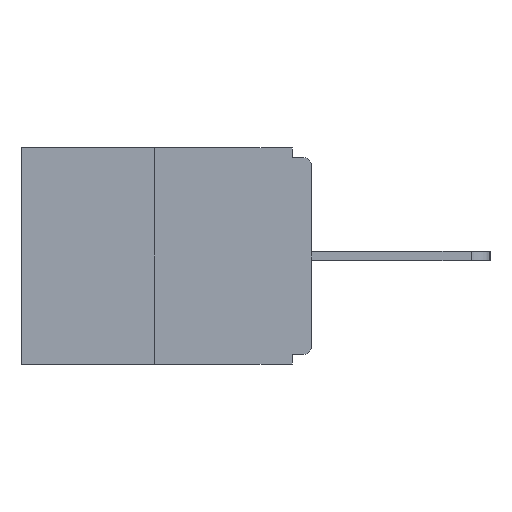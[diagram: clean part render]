
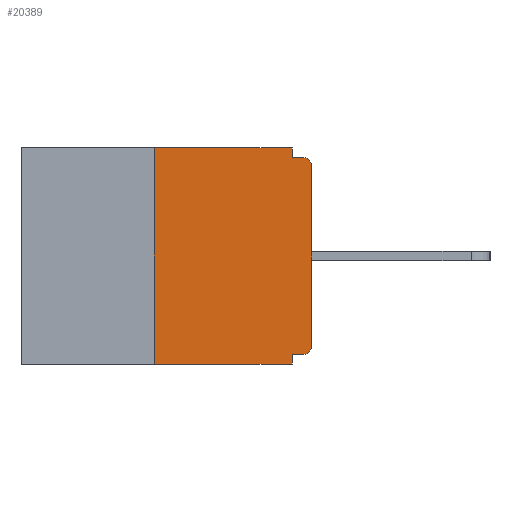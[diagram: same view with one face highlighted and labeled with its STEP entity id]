
A CAD part, left-side view. The second image highlights one B-rep face of the part: STEP entity #20389.
In plain terms, the highlighted planar face has unit normal (-1, 0, 0).
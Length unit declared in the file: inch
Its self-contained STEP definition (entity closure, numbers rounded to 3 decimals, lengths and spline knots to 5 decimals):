
#1220 = VERTEX_POINT ( 'NONE', #17548 ) ;
#1407 = ORIENTED_EDGE ( 'NONE', *, *, #8401, .F. ) ;
#2063 = VERTEX_POINT ( 'NONE', #13509 ) ;
#2719 = VERTEX_POINT ( 'NONE', #18350 ) ;
#2944 = LINE ( 'NONE', #21198, #15774 ) ;
#2949 = DIRECTION ( 'NONE',  ( 0., 0., -1. ) ) ;
#3166 = LINE ( 'NONE', #19771, #17741 ) ;
#3324 = ORIENTED_EDGE ( 'NONE', *, *, #24684, .T. ) ;
#3380 = VERTEX_POINT ( 'NONE', #17262 ) ;
#3836 = PLANE ( 'NONE',  #10884 ) ;
#3865 = EDGE_CURVE ( 'NONE', #14856, #2719, #7147, .T. ) ;
#3969 = DIRECTION ( 'NONE',  ( 0., 0., -1. ) ) ;
#4309 = ORIENTED_EDGE ( 'NONE', *, *, #19632, .F. ) ;
#4408 = ORIENTED_EDGE ( 'NONE', *, *, #24404, .F. ) ;
#4678 = ORIENTED_EDGE ( 'NONE', *, *, #18604, .T. ) ;
#4905 = EDGE_CURVE ( 'NONE', #25087, #2719, #6187, .T. ) ;
#5219 = CARTESIAN_POINT ( 'NONE',  ( 0., 0.46, -0.343 ) ) ;
#6042 = DIRECTION ( 'NONE',  ( 0., 0., -1. ) ) ;
#6187 = LINE ( 'NONE', #24744, #19997 ) ;
#6413 = ORIENTED_EDGE ( 'NONE', *, *, #9980, .F. ) ;
#7147 = LINE ( 'NONE', #5219, #26081 ) ;
#7613 = LINE ( 'NONE', #7879, #17955 ) ;
#7879 = CARTESIAN_POINT ( 'NONE',  ( 0., 0.25, 0. ) ) ;
#8017 = DIRECTION ( 'NONE',  ( 0., 0., 1. ) ) ;
#8219 = VERTEX_POINT ( 'NONE', #12792 ) ;
#8401 = EDGE_CURVE ( 'NONE', #1220, #25087, #2944, .T. ) ;
#9290 = CARTESIAN_POINT ( 'NONE',  ( 0., 0.015, -0.03 ) ) ;
#9309 = CARTESIAN_POINT ( 'NONE',  ( 0., 0.015, -0.015 ) ) ;
#9608 = LINE ( 'NONE', #24181, #14221 ) ;
#9980 = EDGE_CURVE ( 'NONE', #3380, #2063, #12893, .T. ) ;
#10155 = AXIS2_PLACEMENT_3D ( 'NONE', #17661, #19696, #2949 ) ;
#10222 = ORIENTED_EDGE ( 'NONE', *, *, #20641, .T. ) ;
#10619 = VECTOR ( 'NONE', #19005, 39.37008 ) ;
#10884 = AXIS2_PLACEMENT_3D ( 'NONE', #22901, #12428, #3969 ) ;
#10906 = CIRCLE ( 'NONE', #26132, 0.015 ) ;
#11324 = DIRECTION ( 'NONE',  ( -1., 0., 0. ) ) ;
#12428 = DIRECTION ( 'NONE',  ( 1., 0., 0. ) ) ;
#12792 = CARTESIAN_POINT ( 'NONE',  ( 0., 0., -0.03 ) ) ;
#12850 = EDGE_LOOP ( 'NONE', ( #6413, #4408, #17212, #13852, #1407, #3324, #4678, #10222, #20142, #4309 ) ) ;
#12893 = LINE ( 'NONE', #18222, #10619 ) ;
#13036 = VECTOR ( 'NONE', #21183, 39.37008 ) ;
#13501 = DIRECTION ( 'NONE',  ( 0., 0., -1. ) ) ;
#13509 = CARTESIAN_POINT ( 'NONE',  ( 0., 0.031, 0. ) ) ;
#13852 = ORIENTED_EDGE ( 'NONE', *, *, #4905, .F. ) ;
#14221 = VECTOR ( 'NONE', #26626, 39.37008 ) ;
#14856 = VERTEX_POINT ( 'NONE', #17144 ) ;
#15366 = DIRECTION ( 'NONE',  ( 0., 1., 0. ) ) ;
#15774 = VECTOR ( 'NONE', #15366, 39.37008 ) ;
#16039 = VERTEX_POINT ( 'NONE', #17068 ) ;
#16088 = VERTEX_POINT ( 'NONE', #9309 ) ;
#17068 = CARTESIAN_POINT ( 'NONE',  ( 0., 0.031, -0.015 ) ) ;
#17132 = EDGE_CURVE ( 'NONE', #16039, #16088, #9608, .T. ) ;
#17144 = CARTESIAN_POINT ( 'NONE',  ( 0., 0.25, -0.343 ) ) ;
#17212 = ORIENTED_EDGE ( 'NONE', *, *, #3865, .T. ) ;
#17262 = CARTESIAN_POINT ( 'NONE',  ( 0., 0.25, 0. ) ) ;
#17548 = CARTESIAN_POINT ( 'NONE',  ( 0., 0.015, -0.328 ) ) ;
#17661 = CARTESIAN_POINT ( 'NONE',  ( 0., 0.015, -0.313 ) ) ;
#17741 = VECTOR ( 'NONE', #25526, 39.37008 ) ;
#17955 = VECTOR ( 'NONE', #8017, 39.37008 ) ;
#18222 = CARTESIAN_POINT ( 'NONE',  ( 0., 0.46, 0. ) ) ;
#18350 = CARTESIAN_POINT ( 'NONE',  ( 0., 0.031, -0.343 ) ) ;
#18604 = EDGE_CURVE ( 'NONE', #21990, #8219, #3166, .T. ) ;
#18827 = CIRCLE ( 'NONE', #10155, 0.015 ) ;
#19005 = DIRECTION ( 'NONE',  ( 0., -1., 0. ) ) ;
#19632 = EDGE_CURVE ( 'NONE', #2063, #16039, #23514, .T. ) ;
#19696 = DIRECTION ( 'NONE',  ( -1., 0., 0. ) ) ;
#19771 = CARTESIAN_POINT ( 'NONE',  ( 0., 0., 0. ) ) ;
#19997 = VECTOR ( 'NONE', #6042, 39.37008 ) ;
#20142 = ORIENTED_EDGE ( 'NONE', *, *, #17132, .F. ) ;
#20389 = ADVANCED_FACE ( 'NONE', ( #22497 ), #3836, .F. ) ;
#20641 = EDGE_CURVE ( 'NONE', #8219, #16088, #10906, .T. ) ;
#21183 = DIRECTION ( 'NONE',  ( 0., 0., -1. ) ) ;
#21198 = CARTESIAN_POINT ( 'NONE',  ( 0., 0., -0.328 ) ) ;
#21706 = DIRECTION ( 'NONE',  ( 0., -1., 0. ) ) ;
#21990 = VERTEX_POINT ( 'NONE', #26832 ) ;
#22497 = FACE_OUTER_BOUND ( 'NONE', #12850, .T. ) ;
#22901 = CARTESIAN_POINT ( 'NONE',  ( 0., 0.46, 0. ) ) ;
#23514 = LINE ( 'NONE', #25840, #13036 ) ;
#24181 = CARTESIAN_POINT ( 'NONE',  ( 0., 0., -0.015 ) ) ;
#24404 = EDGE_CURVE ( 'NONE', #14856, #3380, #7613, .T. ) ;
#24684 = EDGE_CURVE ( 'NONE', #1220, #21990, #18827, .T. ) ;
#24744 = CARTESIAN_POINT ( 'NONE',  ( 0., 0.031, -0.343 ) ) ;
#25087 = VERTEX_POINT ( 'NONE', #26906 ) ;
#25526 = DIRECTION ( 'NONE',  ( 0., 0., 1. ) ) ;
#25840 = CARTESIAN_POINT ( 'NONE',  ( 0., 0.031, 0. ) ) ;
#26081 = VECTOR ( 'NONE', #21706, 39.37008 ) ;
#26132 = AXIS2_PLACEMENT_3D ( 'NONE', #9290, #11324, #13501 ) ;
#26626 = DIRECTION ( 'NONE',  ( 0., -1., 0. ) ) ;
#26832 = CARTESIAN_POINT ( 'NONE',  ( 0., 0., -0.313 ) ) ;
#26906 = CARTESIAN_POINT ( 'NONE',  ( 0., 0.031, -0.328 ) ) ;
